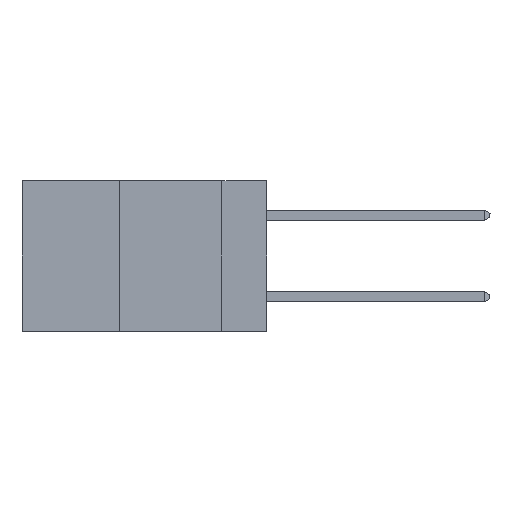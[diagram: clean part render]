
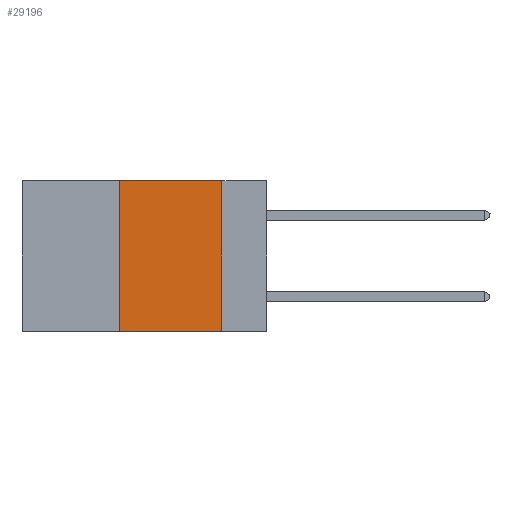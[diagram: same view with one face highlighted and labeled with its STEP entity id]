
A CAD part, left-side view. The second image highlights one B-rep face of the part: STEP entity #29196.
In plain terms, the highlighted planar face has unit normal (-1, 0, 0).
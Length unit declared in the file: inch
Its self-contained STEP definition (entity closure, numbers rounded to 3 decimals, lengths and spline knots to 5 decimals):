
#491 = CARTESIAN_POINT ( 'NONE',  ( 0., 0.36, 0. ) ) ;
#2804 = CARTESIAN_POINT ( 'NONE',  ( 0., 0.11, 0. ) ) ;
#2812 = CARTESIAN_POINT ( 'NONE',  ( 0., 0.36, -0.37 ) ) ;
#3374 = VECTOR ( 'NONE', #31735, 39.37008 ) ;
#3943 = VECTOR ( 'NONE', #5533, 39.37008 ) ;
#4840 = DIRECTION ( 'NONE',  ( 1., 0., 0. ) ) ;
#5533 = DIRECTION ( 'NONE',  ( 0., 0., -1. ) ) ;
#6987 = DIRECTION ( 'NONE',  ( 0., -1., 0. ) ) ;
#7552 = PLANE ( 'NONE',  #7787 ) ;
#7787 = AXIS2_PLACEMENT_3D ( 'NONE', #15521, #4840, #25711 ) ;
#9537 = CARTESIAN_POINT ( 'NONE',  ( 0., 0.6, -0.37 ) ) ;
#9709 = ORIENTED_EDGE ( 'NONE', *, *, #23133, .F. ) ;
#10368 = VERTEX_POINT ( 'NONE', #10427 ) ;
#10427 = CARTESIAN_POINT ( 'NONE',  ( 0., 0.11, -0.37 ) ) ;
#11506 = VERTEX_POINT ( 'NONE', #12199 ) ;
#11580 = LINE ( 'NONE', #9537, #29437 ) ;
#12199 = CARTESIAN_POINT ( 'NONE',  ( 0., 0.36, 0. ) ) ;
#12475 = FACE_OUTER_BOUND ( 'NONE', #23245, .T. ) ;
#13402 = LINE ( 'NONE', #491, #3374 ) ;
#15521 = CARTESIAN_POINT ( 'NONE',  ( 0., 0.6, 0. ) ) ;
#15774 = EDGE_CURVE ( 'NONE', #11506, #28790, #23680, .T. ) ;
#20156 = EDGE_CURVE ( 'NONE', #30041, #11506, #13402, .T. ) ;
#20324 = CARTESIAN_POINT ( 'NONE',  ( 0., 0.11, 0. ) ) ;
#21312 = DIRECTION ( 'NONE',  ( 0., -1., 0. ) ) ;
#21646 = CARTESIAN_POINT ( 'NONE',  ( 0., 0.6, 0. ) ) ;
#23133 = EDGE_CURVE ( 'NONE', #28790, #10368, #26070, .T. ) ;
#23245 = EDGE_LOOP ( 'NONE', ( #9709, #25689, #25114, #29871 ) ) ;
#23253 = VECTOR ( 'NONE', #21312, 39.37008 ) ;
#23680 = LINE ( 'NONE', #21646, #23253 ) ;
#23804 = EDGE_CURVE ( 'NONE', #30041, #10368, #11580, .T. ) ;
#25114 = ORIENTED_EDGE ( 'NONE', *, *, #20156, .F. ) ;
#25689 = ORIENTED_EDGE ( 'NONE', *, *, #15774, .F. ) ;
#25711 = DIRECTION ( 'NONE',  ( 0., 0., -1. ) ) ;
#26070 = LINE ( 'NONE', #2804, #3943 ) ;
#28790 = VERTEX_POINT ( 'NONE', #20324 ) ;
#29196 = ADVANCED_FACE ( 'NONE', ( #12475 ), #7552, .F. ) ;
#29437 = VECTOR ( 'NONE', #6987, 39.37008 ) ;
#29871 = ORIENTED_EDGE ( 'NONE', *, *, #23804, .T. ) ;
#30041 = VERTEX_POINT ( 'NONE', #2812 ) ;
#31735 = DIRECTION ( 'NONE',  ( 0., 0., 1. ) ) ;
